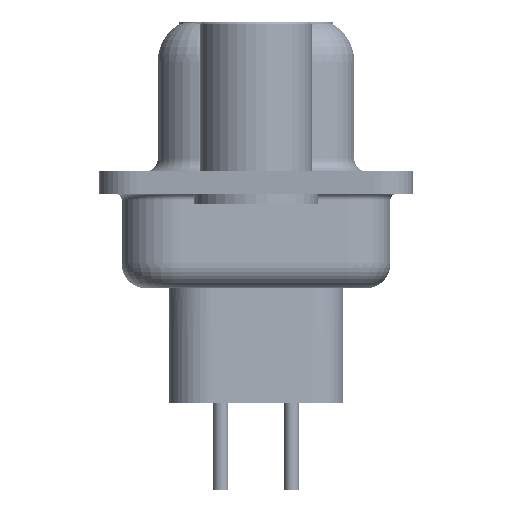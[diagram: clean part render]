
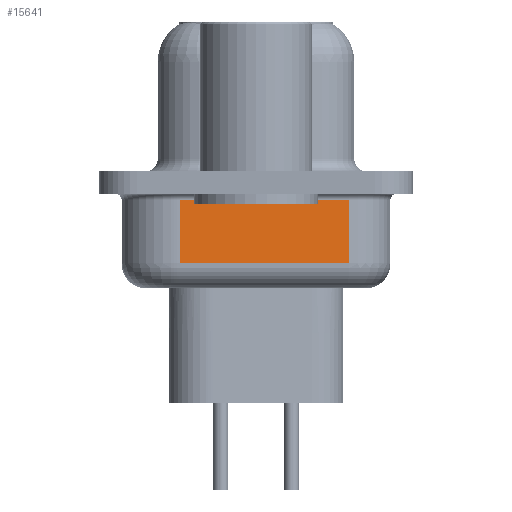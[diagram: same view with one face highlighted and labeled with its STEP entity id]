
A CAD part, left-side view. The second image highlights one B-rep face of the part: STEP entity #15641.
In plain terms, the highlighted planar face has unit normal (-0.985, -0.174, 0).
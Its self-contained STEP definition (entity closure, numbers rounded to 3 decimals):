
#607 = LINE ( 'NONE', #24357, #15785 ) ;
#1098 = DIRECTION ( 'NONE',  ( 0.985, 0.174, 0. ) ) ;
#1242 = ORIENTED_EDGE ( 'NONE', *, *, #4340, .T. ) ;
#4184 = DIRECTION ( 'NONE',  ( 0., 0., 1. ) ) ;
#4208 = ORIENTED_EDGE ( 'NONE', *, *, #15466, .T. ) ;
#4272 = CARTESIAN_POINT ( 'NONE',  ( 4.049, -3.747, -3.25 ) ) ;
#4340 = EDGE_CURVE ( 'NONE', #7658, #19895, #607, .T. ) ;
#4555 = CARTESIAN_POINT ( 'NONE',  ( 4.049, -3.747, -0.7 ) ) ;
#7658 = VERTEX_POINT ( 'NONE', #20736 ) ;
#8343 = DIRECTION ( 'NONE',  ( -0.174, 0.985, 0. ) ) ;
#9050 = VECTOR ( 'NONE', #19680, 1000. ) ;
#10089 = CARTESIAN_POINT ( 'NONE',  ( 4.049, -3.747, -4.25 ) ) ;
#12906 = ORIENTED_EDGE ( 'NONE', *, *, #28032, .T. ) ;
#13073 = FACE_OUTER_BOUND ( 'NONE', #18949, .T. ) ;
#13082 = AXIS2_PLACEMENT_3D ( 'NONE', #20136, #1098, #8343 ) ;
#15466 = EDGE_CURVE ( 'NONE', #19895, #17394, #17498, .T. ) ;
#15641 = ADVANCED_FACE ( 'NONE', ( #13073 ), #27633, .F. ) ;
#15785 = VECTOR ( 'NONE', #29488, 1000. ) ;
#17394 = VERTEX_POINT ( 'NONE', #4555 ) ;
#17498 = LINE ( 'NONE', #10089, #9050 ) ;
#18347 = CARTESIAN_POINT ( 'NONE',  ( 2.85, 3.053, -4.25 ) ) ;
#18949 = EDGE_LOOP ( 'NONE', ( #29709, #1242, #4208, #12906 ) ) ;
#19373 = LINE ( 'NONE', #28894, #23789 ) ;
#19680 = DIRECTION ( 'NONE',  ( 0., 0., 1. ) ) ;
#19895 = VERTEX_POINT ( 'NONE', #4272 ) ;
#20136 = CARTESIAN_POINT ( 'NONE',  ( 2.85, 3.053, -4.25 ) ) ;
#20713 = VECTOR ( 'NONE', #4184, 1000. ) ;
#20736 = CARTESIAN_POINT ( 'NONE',  ( 2.85, 3.053, -3.25 ) ) ;
#23493 = LINE ( 'NONE', #18347, #20713 ) ;
#23789 = VECTOR ( 'NONE', #29040, 1000. ) ;
#24163 = VERTEX_POINT ( 'NONE', #28236 ) ;
#24357 = CARTESIAN_POINT ( 'NONE',  ( 2.85, 3.053, -3.25 ) ) ;
#26724 = EDGE_CURVE ( 'NONE', #7658, #24163, #23493, .T. ) ;
#27633 = PLANE ( 'NONE',  #13082 ) ;
#28032 = EDGE_CURVE ( 'NONE', #17394, #24163, #19373, .T. ) ;
#28236 = CARTESIAN_POINT ( 'NONE',  ( 2.85, 3.053, -0.7 ) ) ;
#28894 = CARTESIAN_POINT ( 'NONE',  ( 2.85, 3.053, -0.7 ) ) ;
#29040 = DIRECTION ( 'NONE',  ( -0.174, 0.985, 0. ) ) ;
#29488 = DIRECTION ( 'NONE',  ( 0.174, -0.985, 0. ) ) ;
#29709 = ORIENTED_EDGE ( 'NONE', *, *, #26724, .F. ) ;
